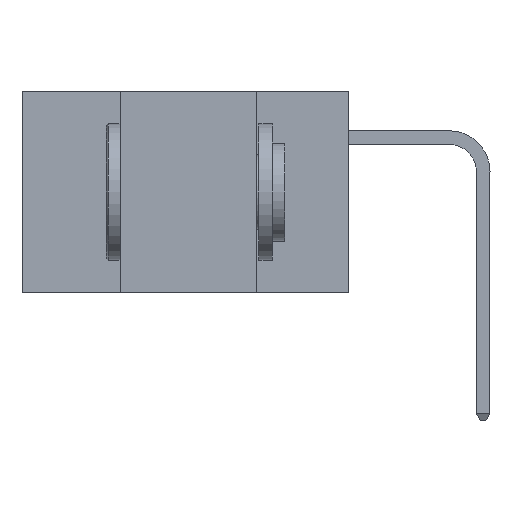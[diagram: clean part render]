
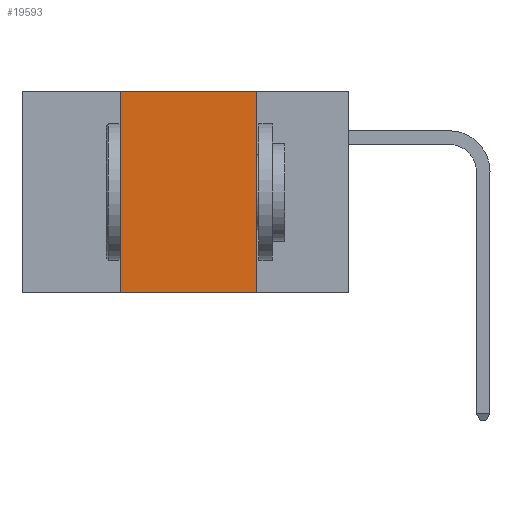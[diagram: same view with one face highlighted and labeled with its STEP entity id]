
A CAD part, left-side view. The second image highlights one B-rep face of the part: STEP entity #19593.
In plain terms, the highlighted planar face has unit normal (-1, 0, 0).
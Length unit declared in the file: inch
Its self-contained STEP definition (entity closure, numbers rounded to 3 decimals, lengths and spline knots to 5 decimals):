
#423 = ORIENTED_EDGE ( 'NONE', *, *, #23827, .F. ) ;
#1295 = CARTESIAN_POINT ( 'NONE',  ( 0., 0.42, -0.37 ) ) ;
#1394 = CARTESIAN_POINT ( 'NONE',  ( 0., 0.6, -0.37 ) ) ;
#1427 = EDGE_CURVE ( 'NONE', #13513, #16415, #23393, .T. ) ;
#2996 = VECTOR ( 'NONE', #13627, 39.37008 ) ;
#3326 = EDGE_CURVE ( 'NONE', #20876, #16415, #19213, .T. ) ;
#5065 = VECTOR ( 'NONE', #7756, 39.37008 ) ;
#5951 = CARTESIAN_POINT ( 'NONE',  ( 0., 0.6, 0. ) ) ;
#6059 = FACE_OUTER_BOUND ( 'NONE', #23255, .T. ) ;
#7756 = DIRECTION ( 'NONE',  ( 0., 0., 1. ) ) ;
#7817 = DIRECTION ( 'NONE',  ( 1., 0., 0. ) ) ;
#8798 = EDGE_CURVE ( 'NONE', #20876, #13814, #21260, .T. ) ;
#9777 = CARTESIAN_POINT ( 'NONE',  ( 0., 0.42, 0. ) ) ;
#10036 = ORIENTED_EDGE ( 'NONE', *, *, #1427, .F. ) ;
#12661 = VECTOR ( 'NONE', #17145, 39.37008 ) ;
#13513 = VERTEX_POINT ( 'NONE', #20927 ) ;
#13627 = DIRECTION ( 'NONE',  ( 0., -1., 0. ) ) ;
#13814 = VERTEX_POINT ( 'NONE', #9777 ) ;
#16112 = CARTESIAN_POINT ( 'NONE',  ( 0., 0.17, -0.37 ) ) ;
#16415 = VERTEX_POINT ( 'NONE', #16112 ) ;
#16690 = ORIENTED_EDGE ( 'NONE', *, *, #8798, .F. ) ;
#17136 = CARTESIAN_POINT ( 'NONE',  ( 0., 0.17, 0. ) ) ;
#17145 = DIRECTION ( 'NONE',  ( 0., 0., -1. ) ) ;
#18326 = VECTOR ( 'NONE', #24203, 39.37008 ) ;
#19213 = LINE ( 'NONE', #1394, #2996 ) ;
#19593 = ADVANCED_FACE ( 'NONE', ( #6059 ), #25922, .F. ) ;
#19874 = CARTESIAN_POINT ( 'NONE',  ( 0., 0.42, 0. ) ) ;
#19931 = AXIS2_PLACEMENT_3D ( 'NONE', #23918, #7817, #21986 ) ;
#20876 = VERTEX_POINT ( 'NONE', #1295 ) ;
#20927 = CARTESIAN_POINT ( 'NONE',  ( 0., 0.17, 0. ) ) ;
#21260 = LINE ( 'NONE', #19874, #5065 ) ;
#21986 = DIRECTION ( 'NONE',  ( 0., 0., -1. ) ) ;
#23255 = EDGE_LOOP ( 'NONE', ( #10036, #423, #16690, #23323 ) ) ;
#23323 = ORIENTED_EDGE ( 'NONE', *, *, #3326, .T. ) ;
#23393 = LINE ( 'NONE', #17136, #12661 ) ;
#23676 = LINE ( 'NONE', #5951, #18326 ) ;
#23827 = EDGE_CURVE ( 'NONE', #13814, #13513, #23676, .T. ) ;
#23918 = CARTESIAN_POINT ( 'NONE',  ( 0., 0.6, 0. ) ) ;
#24203 = DIRECTION ( 'NONE',  ( 0., -1., 0. ) ) ;
#25922 = PLANE ( 'NONE',  #19931 ) ;
